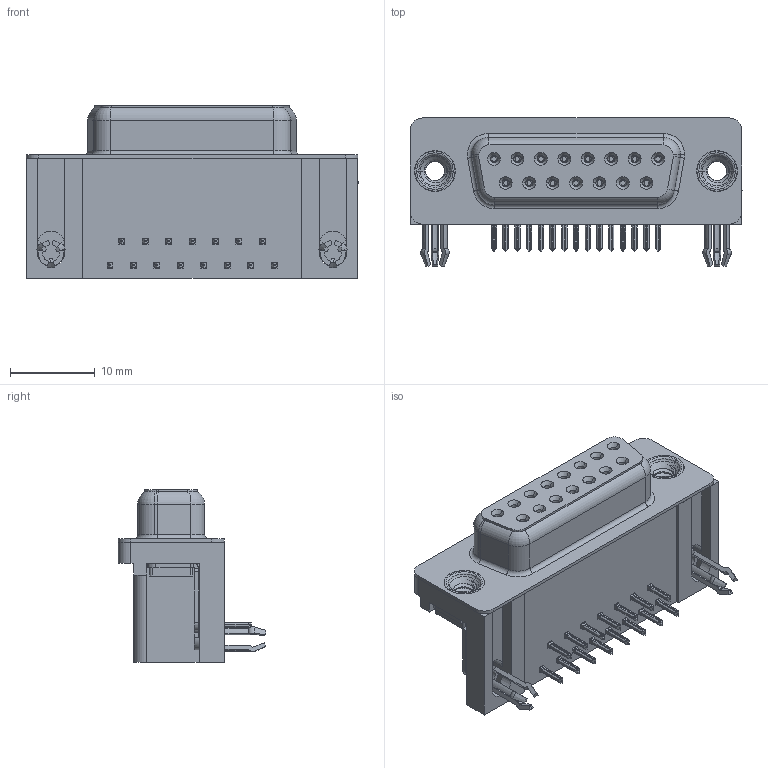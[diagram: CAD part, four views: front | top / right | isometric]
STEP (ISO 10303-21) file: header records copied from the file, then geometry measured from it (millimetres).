
FILE_DESCRIPTION (( 'STEP AP203' ), '1' );
FILE_NAME ('630-015-240-042.STEP', '2021-09-22T13:31:42', ( '' ), ( '' ), 'SwSTEP 2.0', 'SolidWorks 2020', '' );
FILE_SCHEMA (( 'CONFIG_CONTROL_DESIGN' ));
Length unit declared in the file: millimetre
Products named in the file (7): 630 3 Prong Board Lock; 630 4-40 Threaded Rivet; 630-015-240-042; 630 Contact Bottom; 630 Housing_15 Socket; 630 Contact Top; 630 Shell_15 Socket
Assembly tree (21 placements, depth 2):
  630-015-240-042
    630 Housing_15 Socket
    630 Shell_15 Socket
    630 Contact Bottom  x7
    630 Contact Top  x8
    630 3 Prong Board Lock  x2
    630 4-40 Threaded Rivet  x2
Bounding box: 39.22 x 17.48 x 20.4 mm (x, y, z)
Volume: 5869.5 mm3; surface area: 7259.6 mm2
Topology: 21 solids, 21 shells, 2529 faces, 6672 edges, 4200 vertices
Faces by surface type: plane 1110, cylinder 611, bspline 518, cone 228, torus 62
Entity records: 28231 total; most frequent: CARTESIAN_POINT 9291, ORIENTED_EDGE 3840, DIRECTION 3488, EDGE_CURVE 1920, VERTEX_POINT 1226, LINE 1164, VECTOR 1164, AXIS2_PLACEMENT_3D 1162
